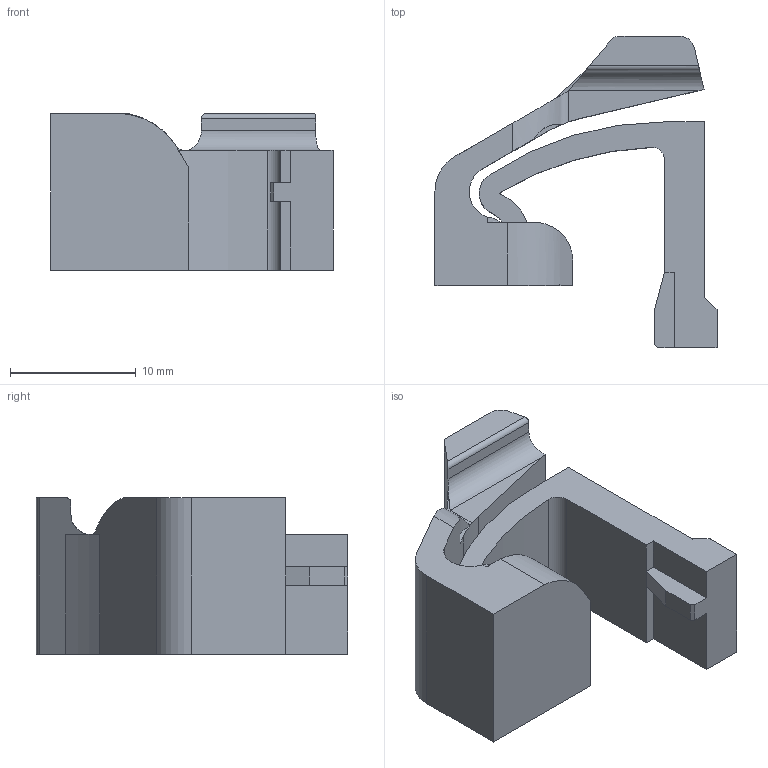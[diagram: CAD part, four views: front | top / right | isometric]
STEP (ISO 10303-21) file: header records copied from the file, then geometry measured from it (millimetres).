
FILE_DESCRIPTION(/* description */ (''),/* implementation_level */ '2;1');
FILE_NAME(/* name */ 'CB High3.stp',/* time_stamp */ '2022-11-09T21:44:06-05:00',/* author */ ('author'),/* organization */ (''),/* preprocessor_version */ 'ST-DEVELOPER v18.1',/* originating_system */ 'Autodesk Inventor 2022',/* authorisation */ '');
FILE_SCHEMA (('AUTOMOTIVE_DESIGN { 1 0 10303 214 3 1 1 }'));
Length unit declared in the file: metre
Products named in the file (1): CB Alt1
Bounding box: 22.42 x 24.74 x 12.45 mm (x, y, z)
Volume: 2430.9 mm3; surface area: 2165.4 mm2
Topology: 1 solids, 1 shells, 58 faces, 164 edges, 109 vertices
Faces by surface type: plane 34, cylinder 24
Entity records: 1970 total; most frequent: CARTESIAN_POINT 365, ORIENTED_EDGE 328, DIRECTION 325, EDGE_CURVE 164, LINE 111, VECTOR 111, VERTEX_POINT 108, AXIS2_PLACEMENT_3D 107
